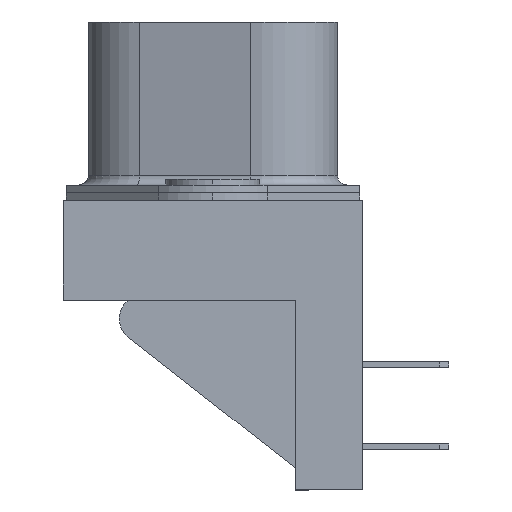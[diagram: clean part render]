
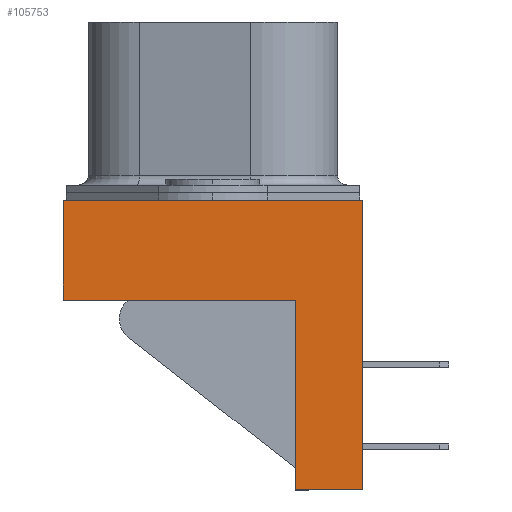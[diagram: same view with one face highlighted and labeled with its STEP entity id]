
A CAD part, left-side view. The second image highlights one B-rep face of the part: STEP entity #105753.
In plain terms, the highlighted planar face has unit normal (-1, 0, 0).
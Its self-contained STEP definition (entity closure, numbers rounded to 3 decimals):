
#1733 = ORIENTED_EDGE ( 'NONE', *, *, #116237, .T. ) ;
#2871 = DIRECTION ( 'NONE',  ( 0., 0., 1. ) ) ;
#4672 = CARTESIAN_POINT ( 'NONE',  ( -4.125, 7.8, -15.1 ) ) ;
#4981 = VECTOR ( 'NONE', #142609, 1000. ) ;
#5737 = ORIENTED_EDGE ( 'NONE', *, *, #152561, .T. ) ;
#6798 = LINE ( 'NONE', #173304, #4981 ) ;
#12428 = DIRECTION ( 'NONE',  ( 0., 1., 0. ) ) ;
#20483 = VECTOR ( 'NONE', #12428, 1000. ) ;
#21790 = ORIENTED_EDGE ( 'NONE', *, *, #119397, .F. ) ;
#23621 = CARTESIAN_POINT ( 'NONE',  ( -4.125, 7.8, -15.1 ) ) ;
#30317 = CARTESIAN_POINT ( 'NONE',  ( -4.125, -4.3, -5.2 ) ) ;
#36309 = LINE ( 'NONE', #23621, #48816 ) ;
#36780 = CARTESIAN_POINT ( 'NONE',  ( -4.125, 7.8, 0. ) ) ;
#40469 = LINE ( 'NONE', #95689, #20483 ) ;
#46379 = LINE ( 'NONE', #145000, #154579 ) ;
#48816 = VECTOR ( 'NONE', #93320, 1000. ) ;
#50037 = VECTOR ( 'NONE', #87311, 1000. ) ;
#58285 = FACE_OUTER_BOUND ( 'NONE', #109781, .T. ) ;
#60547 = ORIENTED_EDGE ( 'NONE', *, *, #86388, .F. ) ;
#63484 = DIRECTION ( 'NONE',  ( 0., -1., 0. ) ) ;
#70086 = DIRECTION ( 'NONE',  ( -1., 0., 0. ) ) ;
#79493 = EDGE_CURVE ( 'NONE', #161576, #137271, #46379, .T. ) ;
#81339 = ORIENTED_EDGE ( 'NONE', *, *, #171418, .F. ) ;
#86388 = EDGE_CURVE ( 'NONE', #89113, #161576, #100617, .T. ) ;
#87311 = DIRECTION ( 'NONE',  ( 0., 0., 1. ) ) ;
#89113 = VERTEX_POINT ( 'NONE', #177993 ) ;
#93320 = DIRECTION ( 'NONE',  ( 0., -1., 0. ) ) ;
#95689 = CARTESIAN_POINT ( 'NONE',  ( -4.125, 7.8, -5.2 ) ) ;
#98138 = DIRECTION ( 'NONE',  ( 0., -1., 0. ) ) ;
#100617 = LINE ( 'NONE', #4672, #115976 ) ;
#105753 = ADVANCED_FACE ( 'NONE', ( #58285 ), #138901, .T. ) ;
#108629 = VERTEX_POINT ( 'NONE', #30317 ) ;
#109781 = EDGE_LOOP ( 'NONE', ( #81339, #21790, #1733, #5737, #168124, #60547 ) ) ;
#115976 = VECTOR ( 'NONE', #2871, 1000. ) ;
#116237 = EDGE_CURVE ( 'NONE', #118915, #163320, #36309, .T. ) ;
#118915 = VERTEX_POINT ( 'NONE', #139177 ) ;
#119397 = EDGE_CURVE ( 'NONE', #118915, #108629, #143439, .T. ) ;
#137139 = CARTESIAN_POINT ( 'NONE',  ( -4.125, 7.8, -15.1 ) ) ;
#137271 = VERTEX_POINT ( 'NONE', #149087 ) ;
#138901 = PLANE ( 'NONE',  #159626 ) ;
#139177 = CARTESIAN_POINT ( 'NONE',  ( -4.125, -4.3, -15.1 ) ) ;
#142609 = DIRECTION ( 'NONE',  ( 0., 0., 1. ) ) ;
#143439 = LINE ( 'NONE', #158775, #50037 ) ;
#145000 = CARTESIAN_POINT ( 'NONE',  ( -4.125, 7.8, 0. ) ) ;
#149087 = CARTESIAN_POINT ( 'NONE',  ( -4.125, -7.8, 0. ) ) ;
#152561 = EDGE_CURVE ( 'NONE', #163320, #137271, #6798, .T. ) ;
#154134 = CARTESIAN_POINT ( 'NONE',  ( -4.125, -7.8, -15.1 ) ) ;
#154579 = VECTOR ( 'NONE', #63484, 1000. ) ;
#158775 = CARTESIAN_POINT ( 'NONE',  ( -4.125, -4.3, -15.1 ) ) ;
#159626 = AXIS2_PLACEMENT_3D ( 'NONE', #137139, #70086, #98138 ) ;
#161576 = VERTEX_POINT ( 'NONE', #36780 ) ;
#163320 = VERTEX_POINT ( 'NONE', #154134 ) ;
#168124 = ORIENTED_EDGE ( 'NONE', *, *, #79493, .F. ) ;
#171418 = EDGE_CURVE ( 'NONE', #108629, #89113, #40469, .T. ) ;
#173304 = CARTESIAN_POINT ( 'NONE',  ( -4.125, -7.8, -15.1 ) ) ;
#177993 = CARTESIAN_POINT ( 'NONE',  ( -4.125, 7.8, -5.2 ) ) ;
